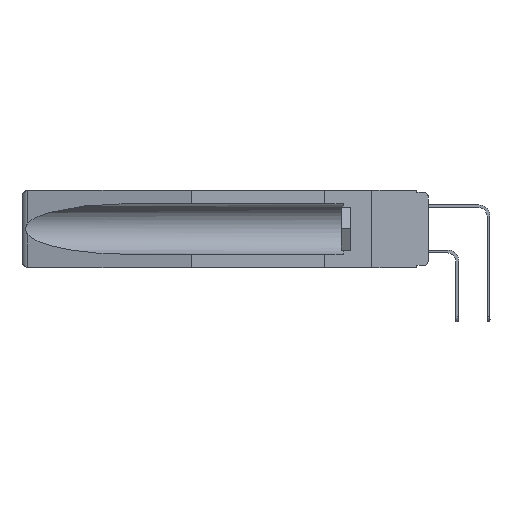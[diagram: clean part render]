
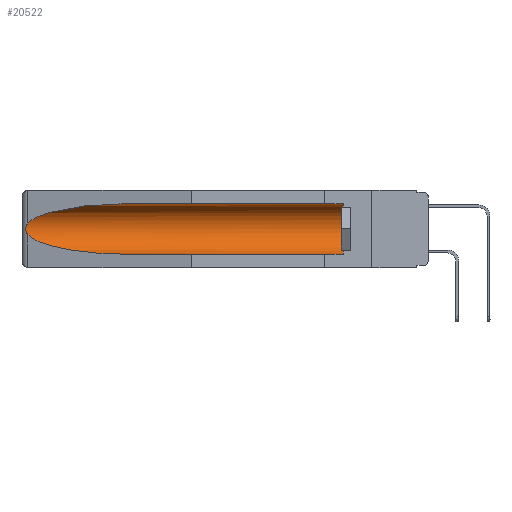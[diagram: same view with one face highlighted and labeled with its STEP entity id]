
A CAD part, left-side view. The second image highlights one B-rep face of the part: STEP entity #20522.
In plain terms, the highlighted cylindrical face has radius 2.857 mm (diameter 5.715 mm), a partial arc.
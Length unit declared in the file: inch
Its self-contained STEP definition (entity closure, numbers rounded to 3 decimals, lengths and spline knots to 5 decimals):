
#533 = CARTESIAN_POINT ( 'NONE',  ( 0.2675, 1.53308, -0.17534 ) ) ;
#936 = CARTESIAN_POINT ( 'NONE',  ( 0.155, 1.07973, -0.059 ) ) ;
#2154 = CARTESIAN_POINT ( 'NONE',  ( 0.26537, 1.52718, -0.14972 ) ) ;
#2532 = AXIS2_PLACEMENT_3D ( 'NONE', #21515, #9184, #4228 ) ;
#2543 = CARTESIAN_POINT ( 'NONE',  ( 0.26537, 1.52718, -0.19328 ) ) ;
#2871 = CIRCLE ( 'NONE', #2532, 0.1125 ) ;
#3190 = ORIENTED_EDGE ( 'NONE', *, *, #9901, .T. ) ;
#3518 = CARTESIAN_POINT ( 'NONE',  ( 0.21114, 1.30732, -0.284 ) ) ;
#3556 = VECTOR ( 'NONE', #4973, 39.37008 ) ;
#4007 = VERTEX_POINT ( 'NONE', #6533 ) ;
#4091 = CARTESIAN_POINT ( 'NONE',  ( 0.26537, 1.52718, -0.14972 ) ) ;
#4224 = VERTEX_POINT ( 'NONE', #18363 ) ;
#4228 = DIRECTION ( 'NONE',  ( 0., 0., 1. ) ) ;
#4823 = VERTEX_POINT ( 'NONE', #14369 ) ;
#4973 = DIRECTION ( 'NONE',  ( 0., 1., 0. ) ) ;
#5127 = EDGE_CURVE ( 'NONE', #4224, #17256, #12631, .T. ) ;
#5249 = VECTOR ( 'NONE', #8292, 39.37008 ) ;
#5738 = EDGE_CURVE ( 'NONE', #8588, #4007, #10678, .T. ) ;
#6533 = CARTESIAN_POINT ( 'NONE',  ( 0.155, 1.07973, -0.284 ) ) ;
#7204 = CARTESIAN_POINT ( 'NONE',  ( 0.26537, 1.52718, -0.19328 ) ) ;
#7433 = ORIENTED_EDGE ( 'NONE', *, *, #5738, .F. ) ;
#7476 = ORIENTED_EDGE ( 'NONE', *, *, #10571, .T. ) ;
#7864 = CARTESIAN_POINT ( 'NONE',  ( 0.155, 1.07973, -0.059 ) ) ;
#8217 = CARTESIAN_POINT ( 'NONE',  ( 0.155, -0.30754, -0.059 ) ) ;
#8292 = DIRECTION ( 'NONE',  ( 0., 1., 0. ) ) ;
#8588 = VERTEX_POINT ( 'NONE', #10089 ) ;
#9184 = DIRECTION ( 'NONE',  ( 0., -1., 0. ) ) ;
#9208 = CARTESIAN_POINT ( 'NONE',  ( 0.26654, 1.53092, -0.15636 ) ) ;
#9901 = EDGE_CURVE ( 'NONE', #4823, #10967, #17516, .T. ) ;
#10089 = CARTESIAN_POINT ( 'NONE',  ( 0.155, 0.126, -0.284 ) ) ;
#10571 = EDGE_CURVE ( 'NONE', #17256, #4823, #15411, .T. ) ;
#10678 = LINE ( 'NONE', #19318, #3556 ) ;
#10967 = VERTEX_POINT ( 'NONE', #15937 ) ;
#11088 = CYLINDRICAL_SURFACE ( 'NONE', #19178, 0.1125 ) ;
#12193 = CARTESIAN_POINT ( 'NONE',  ( 0.25451, 1.48313, -0.24835 ) ) ;
#12631 = LINE ( 'NONE', #8217, #5249 ) ;
#13178 = ORIENTED_EDGE ( 'NONE', *, *, #15456, .T. ) ;
#13984 = CARTESIAN_POINT ( 'NONE',  ( 0.155, -0.30754, -0.1715 ) ) ;
#14056 = DIRECTION ( 'NONE',  ( 0., 1., 0. ) ) ;
#14369 = CARTESIAN_POINT ( 'NONE',  ( 0.26537, 1.52718, -0.14972 ) ) ;
#14636 = CARTESIAN_POINT ( 'NONE',  ( 0.21114, 1.30732, -0.059 ) ) ;
#15043 = CARTESIAN_POINT ( 'NONE',  ( 0.2673, 1.53269, -0.17917 ) ) ;
#15411 =( BOUNDED_CURVE ( )  B_SPLINE_CURVE ( 3, ( #7864, #14636, #16410, #4091 ),
 .UNSPECIFIED., .F., .F. ) 
 B_SPLINE_CURVE_WITH_KNOTS ( ( 4, 4 ),
 ( 4.71239, 6.08839 ),
 .UNSPECIFIED. ) 
 CURVE ( )  GEOMETRIC_REPRESENTATION_ITEM ( )  RATIONAL_B_SPLINE_CURVE ( ( 1., 0.848, 0.848, 1. ) ) 
 REPRESENTATION_ITEM ( '' )  );
#15456 = EDGE_CURVE ( 'NONE', #8588, #4224, #2871, .T. ) ;
#15937 = CARTESIAN_POINT ( 'NONE',  ( 0.26537, 1.52718, -0.19328 ) ) ;
#16410 = CARTESIAN_POINT ( 'NONE',  ( 0.25451, 1.48313, -0.09465 ) ) ;
#16674 = FACE_OUTER_BOUND ( 'NONE', #21603, .T. ) ;
#16811 = CARTESIAN_POINT ( 'NONE',  ( 0.26655, 1.53094, -0.18657 ) ) ;
#17256 = VERTEX_POINT ( 'NONE', #936 ) ;
#17516 = B_SPLINE_CURVE_WITH_KNOTS ( 'NONE', 3,
 ( #2154, #21691, #9208, #18109, #19913, #533, #15043, #16811, #20366, #2543 ),
 .UNSPECIFIED., .F., .F.,
 ( 4, 2, 2, 2, 4 ),
 ( 0., 0.00029, 0.00058, 0.00087, 0.00117 ),
 .UNSPECIFIED. ) ;
#18109 = CARTESIAN_POINT ( 'NONE',  ( 0.2673, 1.5327, -0.16383 ) ) ;
#18363 = CARTESIAN_POINT ( 'NONE',  ( 0.155, 0.126, -0.059 ) ) ;
#18530 = ORIENTED_EDGE ( 'NONE', *, *, #20521, .T. ) ;
#19178 = AXIS2_PLACEMENT_3D ( 'NONE', #13984, #14056, #21257 ) ;
#19318 = CARTESIAN_POINT ( 'NONE',  ( 0.155, -0.30754, -0.284 ) ) ;
#19430 = CARTESIAN_POINT ( 'NONE',  ( 0.155, 1.07973, -0.284 ) ) ;
#19913 = CARTESIAN_POINT ( 'NONE',  ( 0.2675, 1.53308, -0.16763 ) ) ;
#20366 = CARTESIAN_POINT ( 'NONE',  ( 0.26597, 1.5296, -0.19026 ) ) ;
#20521 = EDGE_CURVE ( 'NONE', #10967, #4007, #21212, .T. ) ;
#20522 = ADVANCED_FACE ( 'NONE', ( #16674 ), #11088, .F. ) ;
#21212 =( BOUNDED_CURVE ( )  B_SPLINE_CURVE ( 3, ( #7204, #12193, #3518, #19430 ),
 .UNSPECIFIED., .F., .F. ) 
 B_SPLINE_CURVE_WITH_KNOTS ( ( 4, 4 ),
 ( 0.1948, 1.5708 ),
 .UNSPECIFIED. ) 
 CURVE ( )  GEOMETRIC_REPRESENTATION_ITEM ( )  RATIONAL_B_SPLINE_CURVE ( ( 1., 0.848, 0.848, 1. ) ) 
 REPRESENTATION_ITEM ( '' )  );
#21257 = DIRECTION ( 'NONE',  ( 0., 0., 1. ) ) ;
#21312 = ORIENTED_EDGE ( 'NONE', *, *, #5127, .T. ) ;
#21515 = CARTESIAN_POINT ( 'NONE',  ( 0.155, 0.126, -0.1715 ) ) ;
#21603 = EDGE_LOOP ( 'NONE', ( #7476, #3190, #18530, #7433, #13178, #21312 ) ) ;
#21691 = CARTESIAN_POINT ( 'NONE',  ( 0.26597, 1.52961, -0.15275 ) ) ;
